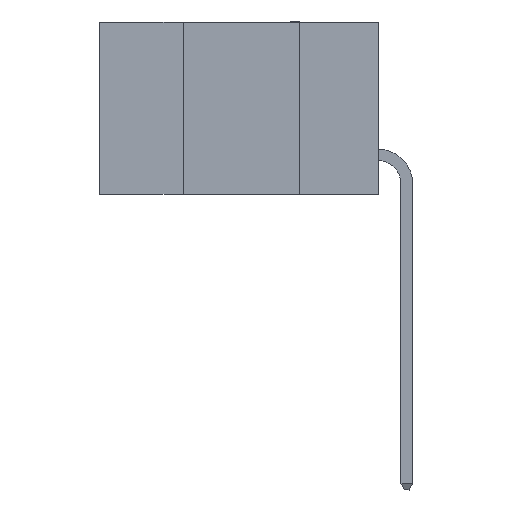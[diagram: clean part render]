
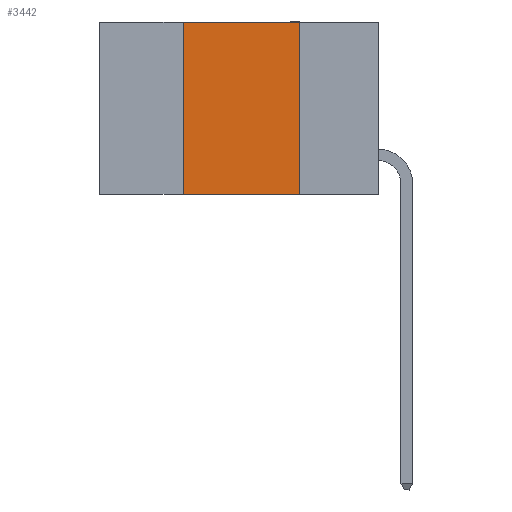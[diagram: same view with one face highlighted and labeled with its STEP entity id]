
A CAD part, left-side view. The second image highlights one B-rep face of the part: STEP entity #3442.
In plain terms, the highlighted planar face has unit normal (-1, 0, 0).
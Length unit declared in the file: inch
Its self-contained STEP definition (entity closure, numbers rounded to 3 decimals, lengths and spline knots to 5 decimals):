
#542 = EDGE_CURVE ( 'NONE', #1974, #11375, #13270, .T. ) ;
#1032 = DIRECTION ( 'NONE',  ( 0., 0., -1. ) ) ;
#1974 = VERTEX_POINT ( 'NONE', #20450 ) ;
#3442 = ADVANCED_FACE ( 'NONE', ( #12130 ), #9111, .F. ) ;
#4113 = DIRECTION ( 'NONE',  ( 0., 0., -1. ) ) ;
#5954 = VECTOR ( 'NONE', #14943, 39.37008 ) ;
#6018 = ORIENTED_EDGE ( 'NONE', *, *, #16091, .T. ) ;
#7139 = CARTESIAN_POINT ( 'NONE',  ( 0., 0.6, 0. ) ) ;
#7662 = LINE ( 'NONE', #12762, #15474 ) ;
#9111 = PLANE ( 'NONE',  #13314 ) ;
#9160 = CARTESIAN_POINT ( 'NONE',  ( 0., 0.17, -0.37 ) ) ;
#9254 = LINE ( 'NONE', #13484, #13052 ) ;
#9910 = CARTESIAN_POINT ( 'NONE',  ( 0., 0.42, 0. ) ) ;
#10178 = ORIENTED_EDGE ( 'NONE', *, *, #14310, .F. ) ;
#10353 = CARTESIAN_POINT ( 'NONE',  ( 0., 0.6, 0. ) ) ;
#11375 = VERTEX_POINT ( 'NONE', #11498 ) ;
#11498 = CARTESIAN_POINT ( 'NONE',  ( 0., 0.42, 0. ) ) ;
#12130 = FACE_OUTER_BOUND ( 'NONE', #19866, .T. ) ;
#12252 = VERTEX_POINT ( 'NONE', #16205 ) ;
#12762 = CARTESIAN_POINT ( 'NONE',  ( 0., 0.17, 0. ) ) ;
#13052 = VECTOR ( 'NONE', #18490, 39.37008 ) ;
#13270 = LINE ( 'NONE', #9910, #5954 ) ;
#13314 = AXIS2_PLACEMENT_3D ( 'NONE', #7139, #21401, #4113 ) ;
#13484 = CARTESIAN_POINT ( 'NONE',  ( 0., 0.6, -0.37 ) ) ;
#14310 = EDGE_CURVE ( 'NONE', #12252, #20319, #7662, .T. ) ;
#14502 = EDGE_CURVE ( 'NONE', #11375, #12252, #21094, .T. ) ;
#14943 = DIRECTION ( 'NONE',  ( 0., 0., 1. ) ) ;
#15474 = VECTOR ( 'NONE', #1032, 39.37008 ) ;
#16091 = EDGE_CURVE ( 'NONE', #1974, #20319, #9254, .T. ) ;
#16205 = CARTESIAN_POINT ( 'NONE',  ( 0., 0.17, 0. ) ) ;
#16302 = ORIENTED_EDGE ( 'NONE', *, *, #542, .F. ) ;
#16319 = VECTOR ( 'NONE', #17126, 39.37008 ) ;
#16546 = ORIENTED_EDGE ( 'NONE', *, *, #14502, .F. ) ;
#17126 = DIRECTION ( 'NONE',  ( 0., -1., 0. ) ) ;
#18490 = DIRECTION ( 'NONE',  ( 0., -1., 0. ) ) ;
#19866 = EDGE_LOOP ( 'NONE', ( #10178, #16546, #16302, #6018 ) ) ;
#20319 = VERTEX_POINT ( 'NONE', #9160 ) ;
#20450 = CARTESIAN_POINT ( 'NONE',  ( 0., 0.42, -0.37 ) ) ;
#21094 = LINE ( 'NONE', #10353, #16319 ) ;
#21401 = DIRECTION ( 'NONE',  ( 1., 0., 0. ) ) ;
